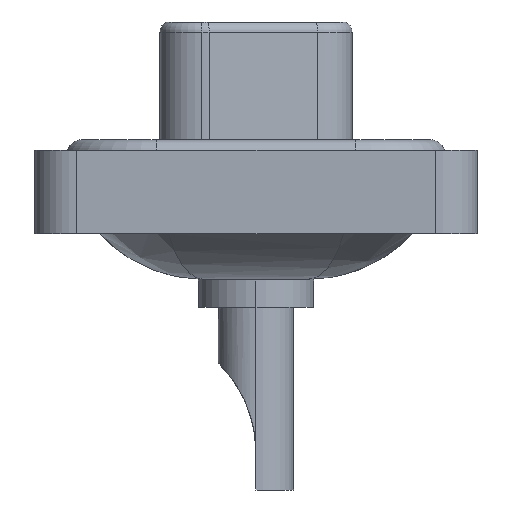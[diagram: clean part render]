
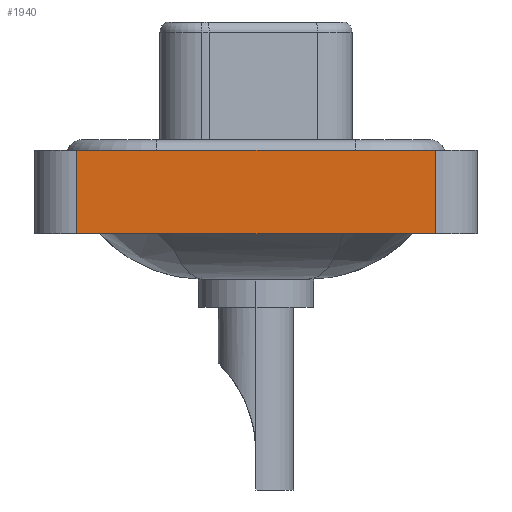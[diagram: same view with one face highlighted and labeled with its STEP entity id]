
A CAD part, left-side view. The second image highlights one B-rep face of the part: STEP entity #1940.
In plain terms, the highlighted planar face has unit normal (-1, 0, 0).
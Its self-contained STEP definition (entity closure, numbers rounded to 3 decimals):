
#192 = EDGE_CURVE ( 'NONE', #10233, #1807, #3546, .T. ) ;
#612 = CARTESIAN_POINT ( 'NONE',  ( -7.25, -8.55, 0.4 ) ) ;
#694 = VECTOR ( 'NONE', #13231, 1000. ) ;
#960 = ORIENTED_EDGE ( 'NONE', *, *, #12332, .F. ) ;
#1236 = DIRECTION ( 'NONE',  ( -1., 0., 0. ) ) ;
#1313 = PLANE ( 'NONE',  #13376 ) ;
#1807 = VERTEX_POINT ( 'NONE', #612 ) ;
#1940 = ADVANCED_FACE ( 'NONE', ( #3511 ), #1313, .T. ) ;
#2218 = CARTESIAN_POINT ( 'NONE',  ( -7.25, -8.55, -3.6 ) ) ;
#2448 = LINE ( 'NONE', #7232, #15487 ) ;
#3511 = FACE_OUTER_BOUND ( 'NONE', #7679, .T. ) ;
#3546 = LINE ( 'NONE', #4816, #694 ) ;
#4816 = CARTESIAN_POINT ( 'NONE',  ( -7.25, -8.55, 0.4 ) ) ;
#4954 = EDGE_CURVE ( 'NONE', #13776, #9815, #11583, .T. ) ;
#6058 = DIRECTION ( 'NONE',  ( 0., 0., 1. ) ) ;
#6765 = ORIENTED_EDGE ( 'NONE', *, *, #192, .F. ) ;
#7232 = CARTESIAN_POINT ( 'NONE',  ( -7.25, 8.55, -3.6 ) ) ;
#7679 = EDGE_LOOP ( 'NONE', ( #13136, #6765, #960, #14703 ) ) ;
#8246 = CARTESIAN_POINT ( 'NONE',  ( -7.25, -8.55, -3.6 ) ) ;
#8471 = DIRECTION ( 'NONE',  ( 0., 0., 1. ) ) ;
#9115 = VECTOR ( 'NONE', #13860, 1000. ) ;
#9815 = VERTEX_POINT ( 'NONE', #8246 ) ;
#10233 = VERTEX_POINT ( 'NONE', #11435 ) ;
#11435 = CARTESIAN_POINT ( 'NONE',  ( -7.25, 8.55, 0.4 ) ) ;
#11583 = LINE ( 'NONE', #14026, #9115 ) ;
#12025 = DIRECTION ( 'NONE',  ( 0., 0., 1. ) ) ;
#12285 = EDGE_CURVE ( 'NONE', #9815, #1807, #12988, .T. ) ;
#12332 = EDGE_CURVE ( 'NONE', #13776, #10233, #2448, .T. ) ;
#12988 = LINE ( 'NONE', #2218, #13216 ) ;
#13136 = ORIENTED_EDGE ( 'NONE', *, *, #12285, .T. ) ;
#13216 = VECTOR ( 'NONE', #6058, 1000. ) ;
#13231 = DIRECTION ( 'NONE',  ( 0., -1., 0. ) ) ;
#13376 = AXIS2_PLACEMENT_3D ( 'NONE', #15564, #1236, #8471 ) ;
#13454 = CARTESIAN_POINT ( 'NONE',  ( -7.25, 8.55, -3.6 ) ) ;
#13776 = VERTEX_POINT ( 'NONE', #13454 ) ;
#13860 = DIRECTION ( 'NONE',  ( 0., -1., 0. ) ) ;
#14026 = CARTESIAN_POINT ( 'NONE',  ( -7.25, -8.55, -3.6 ) ) ;
#14703 = ORIENTED_EDGE ( 'NONE', *, *, #4954, .T. ) ;
#15487 = VECTOR ( 'NONE', #12025, 1000. ) ;
#15564 = CARTESIAN_POINT ( 'NONE',  ( -7.25, -8.55, -3.6 ) ) ;
